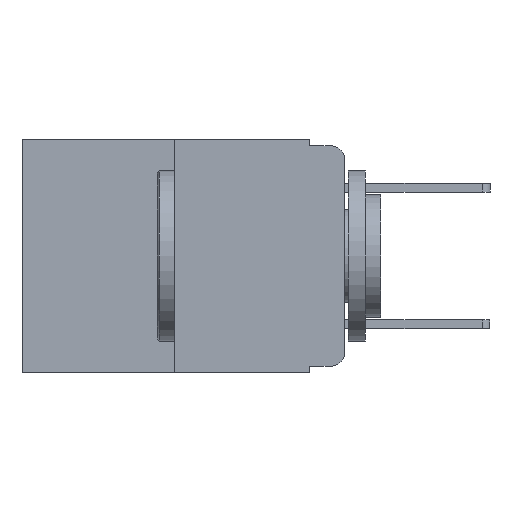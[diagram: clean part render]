
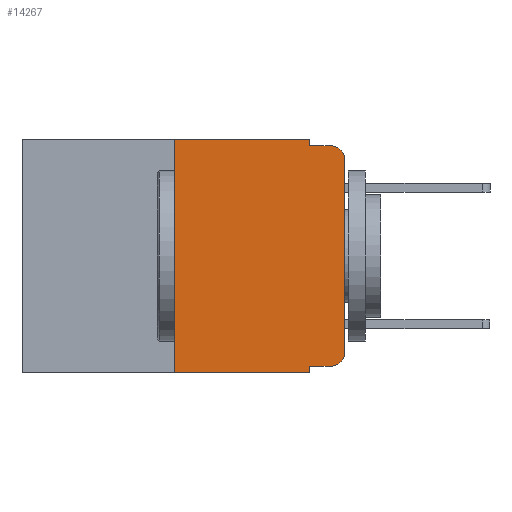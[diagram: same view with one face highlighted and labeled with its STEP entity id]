
A CAD part, left-side view. The second image highlights one B-rep face of the part: STEP entity #14267.
In plain terms, the highlighted planar face has unit normal (-1, 0, 0).
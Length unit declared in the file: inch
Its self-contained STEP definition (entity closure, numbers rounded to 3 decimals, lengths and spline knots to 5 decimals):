
#160 = EDGE_CURVE ( 'NONE', #5865, #2212, #18923, .T. ) ;
#1072 = CARTESIAN_POINT ( 'NONE',  ( 0., 0.051, 0. ) ) ;
#1100 = CARTESIAN_POINT ( 'NONE',  ( 0., 0.02, -0.333 ) ) ;
#1119 = VECTOR ( 'NONE', #6611, 39.37008 ) ;
#1189 = ORIENTED_EDGE ( 'NONE', *, *, #7017, .F. ) ;
#1394 = CARTESIAN_POINT ( 'NONE',  ( 0., 0., 0. ) ) ;
#1395 = AXIS2_PLACEMENT_3D ( 'NONE', #4828, #18934, #6890 ) ;
#1562 = CARTESIAN_POINT ( 'NONE',  ( 0., 0.051, -0.333 ) ) ;
#1813 = ORIENTED_EDGE ( 'NONE', *, *, #3886, .T. ) ;
#2212 = VERTEX_POINT ( 'NONE', #26119 ) ;
#2284 = LINE ( 'NONE', #1394, #23703 ) ;
#2379 = CARTESIAN_POINT ( 'NONE',  ( 0., 0.051, -0.01 ) ) ;
#3136 = ORIENTED_EDGE ( 'NONE', *, *, #160, .F. ) ;
#3728 = DIRECTION ( 'NONE',  ( 0., -1., 0. ) ) ;
#3886 = EDGE_CURVE ( 'NONE', #5741, #12644, #2284, .T. ) ;
#4321 = CARTESIAN_POINT ( 'NONE',  ( 0., 0.051, -0.333 ) ) ;
#4438 = ORIENTED_EDGE ( 'NONE', *, *, #20263, .T. ) ;
#4564 = CARTESIAN_POINT ( 'NONE',  ( 0., 0.051, 0. ) ) ;
#4705 = LINE ( 'NONE', #15922, #26023 ) ;
#4828 = CARTESIAN_POINT ( 'NONE',  ( 0., 0.02, -0.03 ) ) ;
#5337 = DIRECTION ( 'NONE',  ( 0., -1., 0. ) ) ;
#5733 = ORIENTED_EDGE ( 'NONE', *, *, #21695, .T. ) ;
#5741 = VERTEX_POINT ( 'NONE', #15720 ) ;
#5865 = VERTEX_POINT ( 'NONE', #12023 ) ;
#5952 = EDGE_CURVE ( 'NONE', #23560, #5741, #19271, .T. ) ;
#5956 = CARTESIAN_POINT ( 'NONE',  ( 0., 0.25, 0. ) ) ;
#6024 = AXIS2_PLACEMENT_3D ( 'NONE', #11100, #24986, #13111 ) ;
#6307 = DIRECTION ( 'NONE',  ( -1., 0., 0. ) ) ;
#6599 = LINE ( 'NONE', #4564, #1119 ) ;
#6611 = DIRECTION ( 'NONE',  ( 0., 0., -1. ) ) ;
#6890 = DIRECTION ( 'NONE',  ( 0., 0., -1. ) ) ;
#6893 = CIRCLE ( 'NONE', #1395, 0.02 ) ;
#7017 = EDGE_CURVE ( 'NONE', #2212, #25123, #4705, .T. ) ;
#7247 = DIRECTION ( 'NONE',  ( 0., 0., 1. ) ) ;
#8053 = EDGE_CURVE ( 'NONE', #12644, #23868, #6893, .T. ) ;
#8294 = ORIENTED_EDGE ( 'NONE', *, *, #5952, .T. ) ;
#8507 = LINE ( 'NONE', #1562, #13914 ) ;
#9141 = AXIS2_PLACEMENT_3D ( 'NONE', #18373, #6307, #20345 ) ;
#9898 = CARTESIAN_POINT ( 'NONE',  ( 0., 0.051, -0.01 ) ) ;
#10862 = DIRECTION ( 'NONE',  ( 0., 0., 1. ) ) ;
#10895 = CARTESIAN_POINT ( 'NONE',  ( 0., 0.051, 0. ) ) ;
#11100 = CARTESIAN_POINT ( 'NONE',  ( 0., 0.473, 0. ) ) ;
#11164 = EDGE_LOOP ( 'NONE', ( #1813, #12721, #24830, #20801, #1189, #3136, #4438, #15292, #5733, #8294 ) ) ;
#11428 = CARTESIAN_POINT ( 'NONE',  ( 0., 0.473, -0.343 ) ) ;
#12023 = CARTESIAN_POINT ( 'NONE',  ( 0., 0.25, -0.343 ) ) ;
#12644 = VERTEX_POINT ( 'NONE', #20902 ) ;
#12721 = ORIENTED_EDGE ( 'NONE', *, *, #8053, .T. ) ;
#13111 = DIRECTION ( 'NONE',  ( 0., 0., -1. ) ) ;
#13650 = VECTOR ( 'NONE', #7247, 39.37008 ) ;
#13746 = VECTOR ( 'NONE', #19926, 39.37008 ) ;
#13832 = DIRECTION ( 'NONE',  ( 0., -1., 0. ) ) ;
#13914 = VECTOR ( 'NONE', #13832, 39.37008 ) ;
#14267 = ADVANCED_FACE ( 'NONE', ( #14269 ), #22984, .F. ) ;
#14269 = FACE_OUTER_BOUND ( 'NONE', #11164, .T. ) ;
#14379 = VERTEX_POINT ( 'NONE', #25326 ) ;
#15292 = ORIENTED_EDGE ( 'NONE', *, *, #17405, .F. ) ;
#15392 = DIRECTION ( 'NONE',  ( 0., 0., -1. ) ) ;
#15720 = CARTESIAN_POINT ( 'NONE',  ( 0., 0., -0.313 ) ) ;
#15866 = LINE ( 'NONE', #1072, #25139 ) ;
#15922 = CARTESIAN_POINT ( 'NONE',  ( 0., 0.473, 0. ) ) ;
#16325 = CARTESIAN_POINT ( 'NONE',  ( 0., 0.02, -0.01 ) ) ;
#17405 = EDGE_CURVE ( 'NONE', #24493, #14379, #15866, .T. ) ;
#18373 = CARTESIAN_POINT ( 'NONE',  ( 0., 0.02, -0.313 ) ) ;
#18388 = EDGE_CURVE ( 'NONE', #25123, #23337, #6599, .T. ) ;
#18923 = LINE ( 'NONE', #5956, #13650 ) ;
#18934 = DIRECTION ( 'NONE',  ( -1., 0., 0. ) ) ;
#19017 = LINE ( 'NONE', #9898, #13746 ) ;
#19271 = CIRCLE ( 'NONE', #9141, 0.02 ) ;
#19926 = DIRECTION ( 'NONE',  ( 0., -1., 0. ) ) ;
#20020 = VECTOR ( 'NONE', #5337, 39.37008 ) ;
#20263 = EDGE_CURVE ( 'NONE', #5865, #14379, #20628, .T. ) ;
#20345 = DIRECTION ( 'NONE',  ( 0., 0., -1. ) ) ;
#20628 = LINE ( 'NONE', #11428, #20020 ) ;
#20801 = ORIENTED_EDGE ( 'NONE', *, *, #18388, .F. ) ;
#20902 = CARTESIAN_POINT ( 'NONE',  ( 0., 0., -0.03 ) ) ;
#21695 = EDGE_CURVE ( 'NONE', #24493, #23560, #8507, .T. ) ;
#22984 = PLANE ( 'NONE',  #6024 ) ;
#23337 = VERTEX_POINT ( 'NONE', #2379 ) ;
#23560 = VERTEX_POINT ( 'NONE', #1100 ) ;
#23703 = VECTOR ( 'NONE', #10862, 39.37008 ) ;
#23868 = VERTEX_POINT ( 'NONE', #16325 ) ;
#24493 = VERTEX_POINT ( 'NONE', #4321 ) ;
#24830 = ORIENTED_EDGE ( 'NONE', *, *, #25452, .F. ) ;
#24986 = DIRECTION ( 'NONE',  ( 1., 0., 0. ) ) ;
#25123 = VERTEX_POINT ( 'NONE', #10895 ) ;
#25139 = VECTOR ( 'NONE', #15392, 39.37008 ) ;
#25326 = CARTESIAN_POINT ( 'NONE',  ( 0., 0.051, -0.343 ) ) ;
#25452 = EDGE_CURVE ( 'NONE', #23337, #23868, #19017, .T. ) ;
#26023 = VECTOR ( 'NONE', #3728, 39.37008 ) ;
#26119 = CARTESIAN_POINT ( 'NONE',  ( 0., 0.25, 0. ) ) ;
